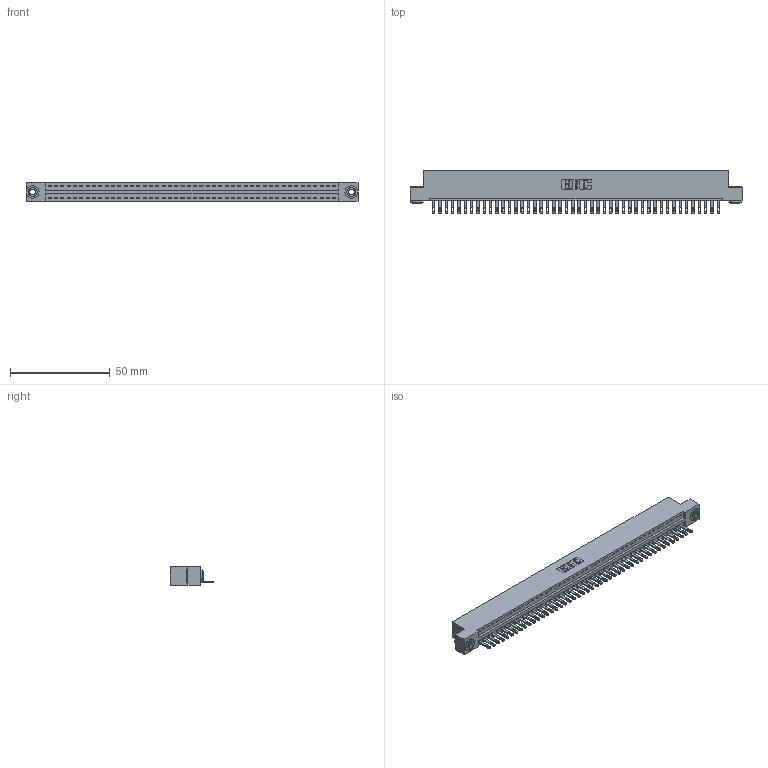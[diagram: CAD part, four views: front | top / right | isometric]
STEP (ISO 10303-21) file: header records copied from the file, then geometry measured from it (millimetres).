
FILE_DESCRIPTION (( 'STEP AP203' ), '1' );
FILE_NAME ('346-046-500-103.STEP', '2022-05-09T19:22:44', ( '' ), ( '' ), 'SwSTEP 2.0', 'SolidWorks 2020', '' );
FILE_SCHEMA (( 'CONFIG_CONTROL_DESIGN' ));
Length unit declared in the file: inch
Products named in the file (4): 345-250-002_345-250-002-102; 345-292-001_345-293-100; 346-046-500-103; 346 Part_Flush Mounting Lugs - 0.156 Dia-TH
Assembly tree (49 placements, depth 2):
  346-046-500-103
    346 Part_Flush Mounting Lugs - 0.156 Dia-TH
    345-292-001_345-293-100  x46
    345-250-002_345-250-002-102  x2
Bounding box: 166.62 x 21.84 x 9.4 mm (x, y, z)
Volume: 16006.9 mm3; surface area: 20408.4 mm2
Topology: 49 solids, 49 shells, 2658 faces, 8169 edges, 5442 vertices
Faces by surface type: plane 1664, cylinder 986, cone 8
Entity records: 29006 total; most frequent: CARTESIAN_POINT 4951, ORIENTED_EDGE 4922, DIRECTION 4395, EDGE_CURVE 2461, LINE 2117, VECTOR 2117, VERTEX_POINT 1638, AXIS2_PLACEMENT_3D 1139
